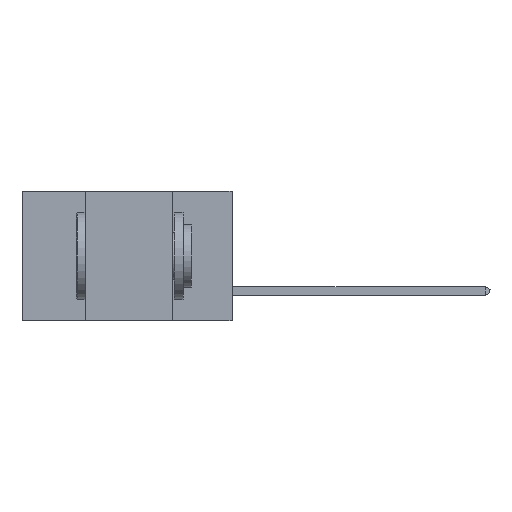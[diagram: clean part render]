
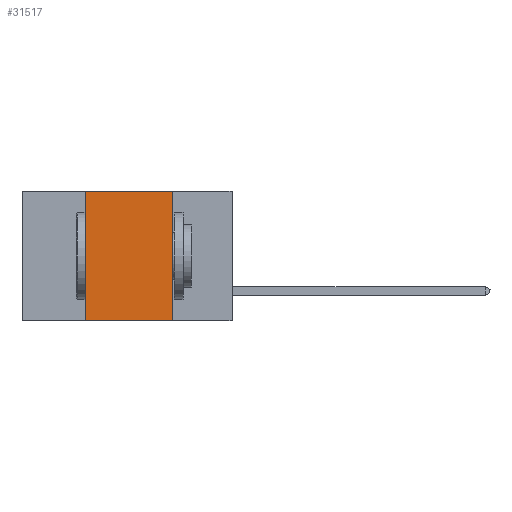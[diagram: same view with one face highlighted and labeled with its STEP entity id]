
A CAD part, left-side view. The second image highlights one B-rep face of the part: STEP entity #31517.
In plain terms, the highlighted planar face has unit normal (-1, 0, 0).
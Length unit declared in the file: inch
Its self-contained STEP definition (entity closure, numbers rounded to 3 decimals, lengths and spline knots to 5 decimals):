
#1410 = AXIS2_PLACEMENT_3D ( 'NONE', #40366, #40530, #18243 ) ;
#2119 = DIRECTION ( 'NONE',  ( 0., 0., 1. ) ) ;
#3935 = EDGE_CURVE ( 'NONE', #20956, #29608, #13974, .T. ) ;
#5846 = EDGE_CURVE ( 'NONE', #16876, #20956, #30689, .T. ) ;
#7786 = ORIENTED_EDGE ( 'NONE', *, *, #5846, .F. ) ;
#10768 = PLANE ( 'NONE',  #1410 ) ;
#12675 = LINE ( 'NONE', #21902, #23700 ) ;
#12756 = VECTOR ( 'NONE', #2119, 39.37008 ) ;
#13974 = LINE ( 'NONE', #25933, #31996 ) ;
#14702 = ORIENTED_EDGE ( 'NONE', *, *, #23223, .T. ) ;
#14915 = DIRECTION ( 'NONE',  ( 0., 0., -1. ) ) ;
#16133 = DIRECTION ( 'NONE',  ( 0., -1., 0. ) ) ;
#16186 = VERTEX_POINT ( 'NONE', #32403 ) ;
#16611 = EDGE_LOOP ( 'NONE', ( #23943, #7786, #17093, #14702 ) ) ;
#16876 = VERTEX_POINT ( 'NONE', #19330 ) ;
#17093 = ORIENTED_EDGE ( 'NONE', *, *, #22466, .F. ) ;
#18243 = DIRECTION ( 'NONE',  ( 0., 0., -1. ) ) ;
#19330 = CARTESIAN_POINT ( 'NONE',  ( 0., 0.42, 0. ) ) ;
#19538 = CARTESIAN_POINT ( 'NONE',  ( 0., 0.6, 0. ) ) ;
#20956 = VERTEX_POINT ( 'NONE', #25720 ) ;
#21881 = FACE_OUTER_BOUND ( 'NONE', #16611, .T. ) ;
#21902 = CARTESIAN_POINT ( 'NONE',  ( 0., 0.6, -0.37 ) ) ;
#22466 = EDGE_CURVE ( 'NONE', #16186, #16876, #30781, .T. ) ;
#23223 = EDGE_CURVE ( 'NONE', #16186, #29608, #12675, .T. ) ;
#23700 = VECTOR ( 'NONE', #43521, 39.37008 ) ;
#23943 = ORIENTED_EDGE ( 'NONE', *, *, #3935, .F. ) ;
#24374 = CARTESIAN_POINT ( 'NONE',  ( 0., 0.42, 0. ) ) ;
#25472 = VECTOR ( 'NONE', #16133, 39.37008 ) ;
#25720 = CARTESIAN_POINT ( 'NONE',  ( 0., 0.17, 0. ) ) ;
#25933 = CARTESIAN_POINT ( 'NONE',  ( 0., 0.17, 0. ) ) ;
#29608 = VERTEX_POINT ( 'NONE', #39450 ) ;
#30689 = LINE ( 'NONE', #19538, #25472 ) ;
#30781 = LINE ( 'NONE', #24374, #12756 ) ;
#31517 = ADVANCED_FACE ( 'NONE', ( #21881 ), #10768, .F. ) ;
#31996 = VECTOR ( 'NONE', #14915, 39.37008 ) ;
#32403 = CARTESIAN_POINT ( 'NONE',  ( 0., 0.42, -0.37 ) ) ;
#39450 = CARTESIAN_POINT ( 'NONE',  ( 0., 0.17, -0.37 ) ) ;
#40366 = CARTESIAN_POINT ( 'NONE',  ( 0., 0.6, 0. ) ) ;
#40530 = DIRECTION ( 'NONE',  ( 1., 0., 0. ) ) ;
#43521 = DIRECTION ( 'NONE',  ( 0., -1., 0. ) ) ;
